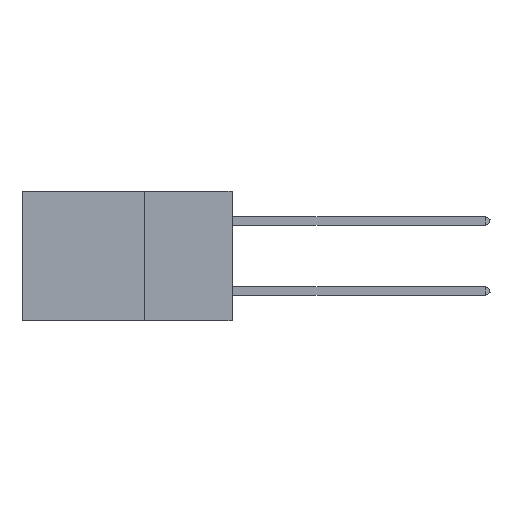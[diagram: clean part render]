
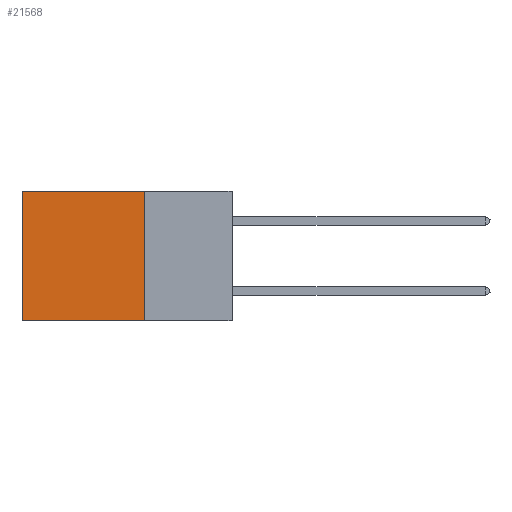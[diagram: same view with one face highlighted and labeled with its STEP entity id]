
A CAD part, left-side view. The second image highlights one B-rep face of the part: STEP entity #21568.
In plain terms, the highlighted planar face has unit normal (-1, 0, 0).
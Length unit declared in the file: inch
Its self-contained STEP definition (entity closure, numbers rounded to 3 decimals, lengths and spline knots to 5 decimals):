
#5 = CARTESIAN_POINT ( 'NONE',  ( 0.2875, 0.25, -0.37 ) ) ;
#836 = VERTEX_POINT ( 'NONE', #28485 ) ;
#1646 = ORIENTED_EDGE ( 'NONE', *, *, #10744, .F. ) ;
#1655 = CARTESIAN_POINT ( 'NONE',  ( 0.2875, 0.25, 0. ) ) ;
#2125 = ORIENTED_EDGE ( 'NONE', *, *, #29937, .T. ) ;
#2277 = CARTESIAN_POINT ( 'NONE',  ( 0.2875, 0.25, -0.37 ) ) ;
#2371 = CARTESIAN_POINT ( 'NONE',  ( 0.2875, 0.25, 0. ) ) ;
#3143 = VECTOR ( 'NONE', #26186, 39.37008 ) ;
#4489 = AXIS2_PLACEMENT_3D ( 'NONE', #24121, #11557, #8828 ) ;
#6053 = EDGE_CURVE ( 'NONE', #25248, #10078, #19759, .T. ) ;
#6262 = DIRECTION ( 'NONE',  ( 0., 1., 0. ) ) ;
#8828 = DIRECTION ( 'NONE',  ( 0., 0., -1. ) ) ;
#9195 = DIRECTION ( 'NONE',  ( 0., 0., -1. ) ) ;
#9393 = VERTEX_POINT ( 'NONE', #28135 ) ;
#10078 = VERTEX_POINT ( 'NONE', #2277 ) ;
#10744 = EDGE_CURVE ( 'NONE', #10078, #836, #16866, .T. ) ;
#11557 = DIRECTION ( 'NONE',  ( 1., 0., 0. ) ) ;
#13649 = VECTOR ( 'NONE', #6262, 39.37008 ) ;
#13656 = FACE_OUTER_BOUND ( 'NONE', #29516, .T. ) ;
#15609 = EDGE_CURVE ( 'NONE', #25248, #9393, #27114, .T. ) ;
#16866 = LINE ( 'NONE', #5, #23380 ) ;
#18429 = CARTESIAN_POINT ( 'NONE',  ( 0.2875, 0.6, 0. ) ) ;
#19241 = CARTESIAN_POINT ( 'NONE',  ( 0.2875, 0.25, 0. ) ) ;
#19759 = LINE ( 'NONE', #1655, #25860 ) ;
#21568 = ADVANCED_FACE ( 'NONE', ( #13656 ), #27177, .F. ) ;
#23380 = VECTOR ( 'NONE', #31344, 39.37008 ) ;
#24121 = CARTESIAN_POINT ( 'NONE',  ( 0.2875, 0.25, 0. ) ) ;
#25248 = VERTEX_POINT ( 'NONE', #2371 ) ;
#25860 = VECTOR ( 'NONE', #9195, 39.37008 ) ;
#26186 = DIRECTION ( 'NONE',  ( 0., 0., -1. ) ) ;
#26333 = ORIENTED_EDGE ( 'NONE', *, *, #15609, .T. ) ;
#27114 = LINE ( 'NONE', #19241, #13649 ) ;
#27177 = PLANE ( 'NONE',  #4489 ) ;
#28135 = CARTESIAN_POINT ( 'NONE',  ( 0.2875, 0.6, 0. ) ) ;
#28485 = CARTESIAN_POINT ( 'NONE',  ( 0.2875, 0.6, -0.37 ) ) ;
#29264 = ORIENTED_EDGE ( 'NONE', *, *, #6053, .F. ) ;
#29516 = EDGE_LOOP ( 'NONE', ( #2125, #1646, #29264, #26333 ) ) ;
#29937 = EDGE_CURVE ( 'NONE', #9393, #836, #30812, .T. ) ;
#30812 = LINE ( 'NONE', #18429, #3143 ) ;
#31344 = DIRECTION ( 'NONE',  ( 0., 1., 0. ) ) ;
